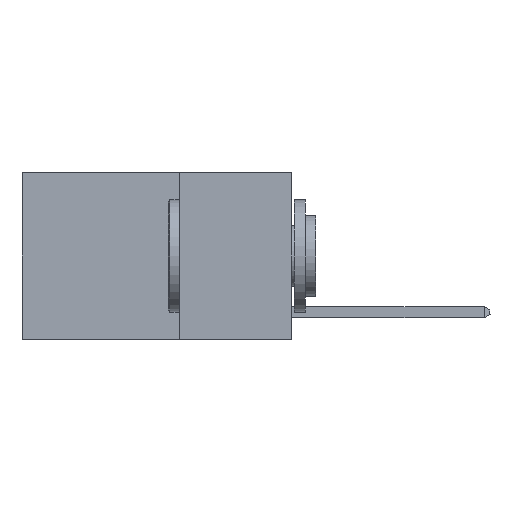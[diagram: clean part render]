
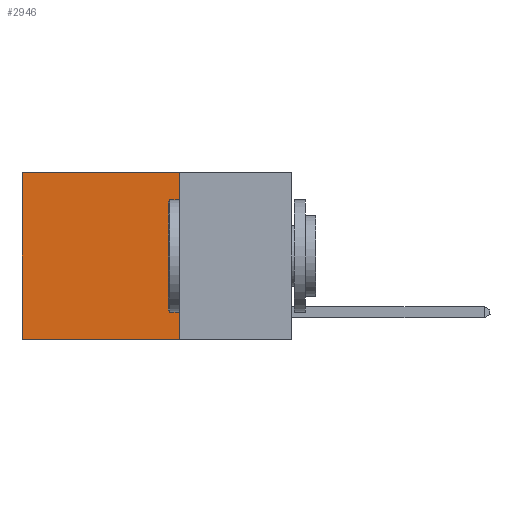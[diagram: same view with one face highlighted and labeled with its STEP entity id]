
A CAD part, left-side view. The second image highlights one B-rep face of the part: STEP entity #2946.
In plain terms, the highlighted planar face has unit normal (-1, 0, 0).
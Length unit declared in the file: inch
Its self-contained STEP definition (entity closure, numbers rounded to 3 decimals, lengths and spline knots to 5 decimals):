
#504 = LINE ( 'NONE', #3603, #9518 ) ;
#1012 = EDGE_CURVE ( 'NONE', #4717, #8597, #1233, .T. ) ;
#1233 = LINE ( 'NONE', #7648, #7938 ) ;
#2582 = CARTESIAN_POINT ( 'NONE',  ( 0.2625, 0.25, 0. ) ) ;
#2946 = ADVANCED_FACE ( 'NONE', ( #10224 ), #4334, .F. ) ;
#3461 = DIRECTION ( 'NONE',  ( 0., 1., 0. ) ) ;
#3514 = VERTEX_POINT ( 'NONE', #7035 ) ;
#3603 = CARTESIAN_POINT ( 'NONE',  ( 0.2625, 0.6, 0. ) ) ;
#4018 = DIRECTION ( 'NONE',  ( 0., 1., 0. ) ) ;
#4269 = DIRECTION ( 'NONE',  ( 0., 0., -1. ) ) ;
#4334 = PLANE ( 'NONE',  #6606 ) ;
#4717 = VERTEX_POINT ( 'NONE', #7269 ) ;
#4807 = EDGE_CURVE ( 'NONE', #4717, #3514, #7748, .T. ) ;
#4857 = CARTESIAN_POINT ( 'NONE',  ( 0.2625, 0.25, -0.37 ) ) ;
#5186 = DIRECTION ( 'NONE',  ( 1., 0., 0. ) ) ;
#5258 = DIRECTION ( 'NONE',  ( 0., 0., -1. ) ) ;
#5319 = CARTESIAN_POINT ( 'NONE',  ( 0.2625, 0.6, 0. ) ) ;
#5947 = CARTESIAN_POINT ( 'NONE',  ( 0.2625, 0.25, 0. ) ) ;
#6502 = VECTOR ( 'NONE', #4018, 39.37008 ) ;
#6542 = VERTEX_POINT ( 'NONE', #8361 ) ;
#6606 = AXIS2_PLACEMENT_3D ( 'NONE', #2582, #5186, #10979 ) ;
#7035 = CARTESIAN_POINT ( 'NONE',  ( 0.2625, 0.25, -0.37 ) ) ;
#7086 = ORIENTED_EDGE ( 'NONE', *, *, #7566, .T. ) ;
#7100 = ORIENTED_EDGE ( 'NONE', *, *, #9498, .F. ) ;
#7122 = ORIENTED_EDGE ( 'NONE', *, *, #4807, .F. ) ;
#7167 = ORIENTED_EDGE ( 'NONE', *, *, #1012, .T. ) ;
#7269 = CARTESIAN_POINT ( 'NONE',  ( 0.2625, 0.25, 0. ) ) ;
#7566 = EDGE_CURVE ( 'NONE', #8597, #6542, #504, .T. ) ;
#7648 = CARTESIAN_POINT ( 'NONE',  ( 0.2625, 0.25, 0. ) ) ;
#7748 = LINE ( 'NONE', #5947, #9694 ) ;
#7938 = VECTOR ( 'NONE', #3461, 39.37008 ) ;
#8361 = CARTESIAN_POINT ( 'NONE',  ( 0.2625, 0.6, -0.37 ) ) ;
#8597 = VERTEX_POINT ( 'NONE', #5319 ) ;
#8701 = LINE ( 'NONE', #4857, #6502 ) ;
#9498 = EDGE_CURVE ( 'NONE', #3514, #6542, #8701, .T. ) ;
#9518 = VECTOR ( 'NONE', #5258, 39.37008 ) ;
#9694 = VECTOR ( 'NONE', #4269, 39.37008 ) ;
#10224 = FACE_OUTER_BOUND ( 'NONE', #11018, .T. ) ;
#10979 = DIRECTION ( 'NONE',  ( 0., 0., -1. ) ) ;
#11018 = EDGE_LOOP ( 'NONE', ( #7086, #7100, #7122, #7167 ) ) ;
